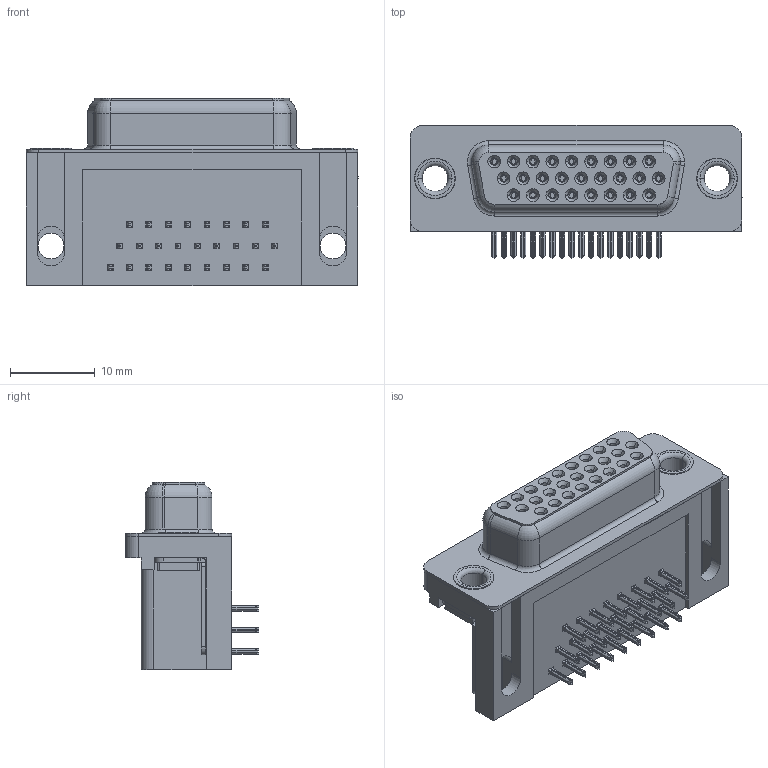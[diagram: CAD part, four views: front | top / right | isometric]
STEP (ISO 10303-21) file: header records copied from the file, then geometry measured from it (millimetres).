
FILE_DESCRIPTION (( 'STEP AP203' ), '1' );
FILE_NAME ('634-026-263-011.STEP', '2018-08-18T02:09:50', ( '' ), ( '' ), 'SwSTEP 2.0', 'SolidWorks 2016', '' );
FILE_SCHEMA (( 'CONFIG_CONTROL_DESIGN' ));
Length unit declared in the file: millimetre
Products named in the file (8): Thru Hole Rivet; 634-026-263-011; 634 Housing_26 Socket; 634 Shell_26 Socket; Contact Bottom; Contact Middle; Contact Top; Thru Hole Board Mount
Assembly tree (32 placements, depth 2):
  634-026-263-011
    634 Housing_26 Socket
    634 Shell_26 Socket
    Contact Bottom  x8
    Contact Middle  x9
    Contact Top  x9
    Thru Hole Board Mount  x2
    Thru Hole Rivet  x2
Bounding box: 39.22 x 15.73 x 22.1 mm (x, y, z)
Volume: 6352.9 mm3; surface area: 9048.3 mm2
Topology: 32 solids, 32 shells, 3939 faces, 10348 edges, 6498 vertices
Faces by surface type: plane 1769, cylinder 920, bspline 904, cone 312, torus 34
Entity records: 34416 total; most frequent: CARTESIAN_POINT 10383, ORIENTED_EDGE 4844, DIRECTION 4315, EDGE_CURVE 2422, VECTOR 1563, LINE 1563, VERTEX_POINT 1542, AXIS2_PLACEMENT_3D 1376
